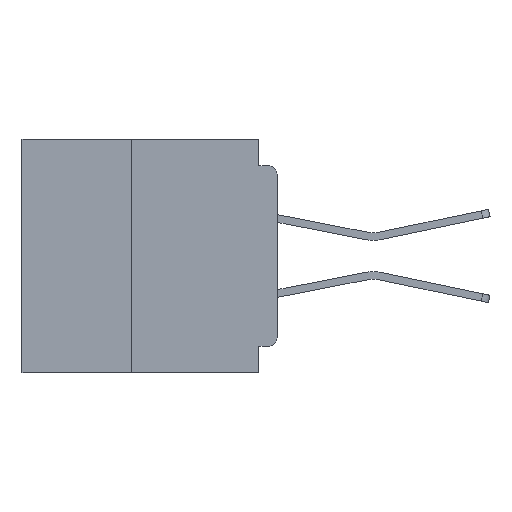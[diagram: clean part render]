
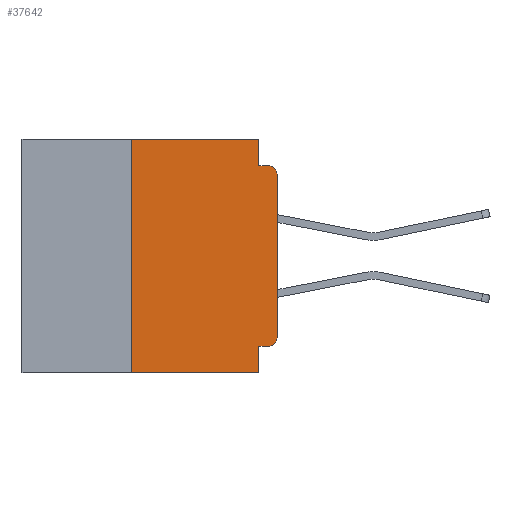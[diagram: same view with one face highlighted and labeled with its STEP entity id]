
A CAD part, left-side view. The second image highlights one B-rep face of the part: STEP entity #37642.
In plain terms, the highlighted planar face has unit normal (-1, 0, 0).
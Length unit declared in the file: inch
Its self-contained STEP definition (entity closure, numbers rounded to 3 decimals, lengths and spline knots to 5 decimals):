
#180 = DIRECTION ( 'NONE',  ( 0., 0., -1. ) ) ;
#420 = EDGE_LOOP ( 'NONE', ( #1617, #32466, #9815, #37045, #18598, #31681, #9294, #14757, #29593, #8314 ) ) ;
#462 = DIRECTION ( 'NONE',  ( -1., 0., 0. ) ) ;
#658 = DIRECTION ( 'NONE',  ( 0., 1., 0. ) ) ;
#1285 = EDGE_CURVE ( 'NONE', #37980, #6313, #38416, .T. ) ;
#1286 = CARTESIAN_POINT ( 'NONE',  ( 0., 0., 0. ) ) ;
#1590 = VERTEX_POINT ( 'NONE', #3400 ) ;
#1617 = ORIENTED_EDGE ( 'NONE', *, *, #13811, .T. ) ;
#2584 = LINE ( 'NONE', #25107, #33942 ) ;
#3364 = CARTESIAN_POINT ( 'NONE',  ( 0., 0.031, -0.355 ) ) ;
#3400 = CARTESIAN_POINT ( 'NONE',  ( 0., 0.031, -0.4 ) ) ;
#4156 = EDGE_CURVE ( 'NONE', #5923, #1590, #33193, .T. ) ;
#4524 = CARTESIAN_POINT ( 'NONE',  ( 0., 0.25, -0.4 ) ) ;
#5350 = VECTOR ( 'NONE', #16878, 39.37008 ) ;
#5704 = EDGE_CURVE ( 'NONE', #22175, #28454, #27125, .T. ) ;
#5923 = VERTEX_POINT ( 'NONE', #15617 ) ;
#6313 = VERTEX_POINT ( 'NONE', #23658 ) ;
#7090 = CARTESIAN_POINT ( 'NONE',  ( 0., 0.015, -0.34 ) ) ;
#8242 = VERTEX_POINT ( 'NONE', #38211 ) ;
#8314 = ORIENTED_EDGE ( 'NONE', *, *, #1285, .T. ) ;
#9245 = DIRECTION ( 'NONE',  ( 0., 0., -1. ) ) ;
#9294 = ORIENTED_EDGE ( 'NONE', *, *, #4156, .T. ) ;
#9815 = ORIENTED_EDGE ( 'NONE', *, *, #5704, .F. ) ;
#10062 = CARTESIAN_POINT ( 'NONE',  ( 0., 0.015, -0.06 ) ) ;
#10334 = LINE ( 'NONE', #27324, #32513 ) ;
#10450 = CARTESIAN_POINT ( 'NONE',  ( 0., 0.437, -0.4 ) ) ;
#11407 = VERTEX_POINT ( 'NONE', #15877 ) ;
#11473 = CARTESIAN_POINT ( 'NONE',  ( 0., 0.437, 0. ) ) ;
#12864 = EDGE_CURVE ( 'NONE', #28240, #1590, #10334, .T. ) ;
#13108 = DIRECTION ( 'NONE',  ( 0., 0., -1. ) ) ;
#13170 = CIRCLE ( 'NONE', #20126, 0.015 ) ;
#13514 = LINE ( 'NONE', #4524, #5350 ) ;
#13811 = EDGE_CURVE ( 'NONE', #6313, #11407, #24458, .T. ) ;
#14183 = LINE ( 'NONE', #25571, #30258 ) ;
#14508 = DIRECTION ( 'NONE',  ( 0., 0., -1. ) ) ;
#14757 = ORIENTED_EDGE ( 'NONE', *, *, #12864, .F. ) ;
#15460 = VECTOR ( 'NONE', #34744, 39.37008 ) ;
#15617 = CARTESIAN_POINT ( 'NONE',  ( 0., 0.25, -0.4 ) ) ;
#15877 = CARTESIAN_POINT ( 'NONE',  ( 0., 0., -0.06 ) ) ;
#16101 = AXIS2_PLACEMENT_3D ( 'NONE', #11473, #32588, #14508 ) ;
#16392 = EDGE_CURVE ( 'NONE', #18901, #8242, #23321, .T. ) ;
#16878 = DIRECTION ( 'NONE',  ( 0., 0., 1. ) ) ;
#18126 = EDGE_CURVE ( 'NONE', #37980, #28240, #2584, .T. ) ;
#18598 = ORIENTED_EDGE ( 'NONE', *, *, #16392, .F. ) ;
#18901 = VERTEX_POINT ( 'NONE', #26232 ) ;
#19440 = DIRECTION ( 'NONE',  ( 0., 0., -1. ) ) ;
#19744 = CARTESIAN_POINT ( 'NONE',  ( 0., 0.015, -0.045 ) ) ;
#20126 = AXIS2_PLACEMENT_3D ( 'NONE', #10062, #31191, #13108 ) ;
#20528 = PLANE ( 'NONE',  #16101 ) ;
#21434 = VECTOR ( 'NONE', #32583, 39.37008 ) ;
#22175 = VERTEX_POINT ( 'NONE', #34175 ) ;
#22669 = DIRECTION ( 'NONE',  ( 0., -1., 0. ) ) ;
#23321 = LINE ( 'NONE', #29564, #21434 ) ;
#23444 = EDGE_CURVE ( 'NONE', #8242, #22175, #14183, .T. ) ;
#23658 = CARTESIAN_POINT ( 'NONE',  ( 0., 0., -0.34 ) ) ;
#24458 = LINE ( 'NONE', #1286, #15460 ) ;
#25107 = CARTESIAN_POINT ( 'NONE',  ( 0., 0., -0.355 ) ) ;
#25571 = CARTESIAN_POINT ( 'NONE',  ( 0., 0.031, 0. ) ) ;
#26232 = CARTESIAN_POINT ( 'NONE',  ( 0., 0.25, 0. ) ) ;
#27125 = LINE ( 'NONE', #35583, #36008 ) ;
#27324 = CARTESIAN_POINT ( 'NONE',  ( 0., 0.031, -0.4 ) ) ;
#28240 = VERTEX_POINT ( 'NONE', #3364 ) ;
#28454 = VERTEX_POINT ( 'NONE', #19744 ) ;
#29564 = CARTESIAN_POINT ( 'NONE',  ( 0., 0.437, 0. ) ) ;
#29593 = ORIENTED_EDGE ( 'NONE', *, *, #18126, .F. ) ;
#30258 = VECTOR ( 'NONE', #19440, 39.37008 ) ;
#31191 = DIRECTION ( 'NONE',  ( -1., 0., 0. ) ) ;
#31233 = AXIS2_PLACEMENT_3D ( 'NONE', #7090, #462, #180 ) ;
#31681 = ORIENTED_EDGE ( 'NONE', *, *, #34854, .F. ) ;
#32259 = VECTOR ( 'NONE', #22669, 39.37008 ) ;
#32466 = ORIENTED_EDGE ( 'NONE', *, *, #33428, .T. ) ;
#32513 = VECTOR ( 'NONE', #9245, 39.37008 ) ;
#32583 = DIRECTION ( 'NONE',  ( 0., -1., 0. ) ) ;
#32588 = DIRECTION ( 'NONE',  ( 1., 0., 0. ) ) ;
#33193 = LINE ( 'NONE', #10450, #32259 ) ;
#33428 = EDGE_CURVE ( 'NONE', #11407, #28454, #13170, .T. ) ;
#33942 = VECTOR ( 'NONE', #658, 39.37008 ) ;
#34121 = CARTESIAN_POINT ( 'NONE',  ( 0., 0.015, -0.355 ) ) ;
#34175 = CARTESIAN_POINT ( 'NONE',  ( 0., 0.031, -0.045 ) ) ;
#34744 = DIRECTION ( 'NONE',  ( 0., 0., 1. ) ) ;
#34854 = EDGE_CURVE ( 'NONE', #5923, #18901, #13514, .T. ) ;
#35583 = CARTESIAN_POINT ( 'NONE',  ( 0., 0., -0.045 ) ) ;
#36008 = VECTOR ( 'NONE', #38542, 39.37008 ) ;
#37045 = ORIENTED_EDGE ( 'NONE', *, *, #23444, .F. ) ;
#37231 = FACE_OUTER_BOUND ( 'NONE', #420, .T. ) ;
#37642 = ADVANCED_FACE ( 'NONE', ( #37231 ), #20528, .F. ) ;
#37980 = VERTEX_POINT ( 'NONE', #34121 ) ;
#38211 = CARTESIAN_POINT ( 'NONE',  ( 0., 0.031, 0. ) ) ;
#38416 = CIRCLE ( 'NONE', #31233, 0.015 ) ;
#38542 = DIRECTION ( 'NONE',  ( 0., -1., 0. ) ) ;
